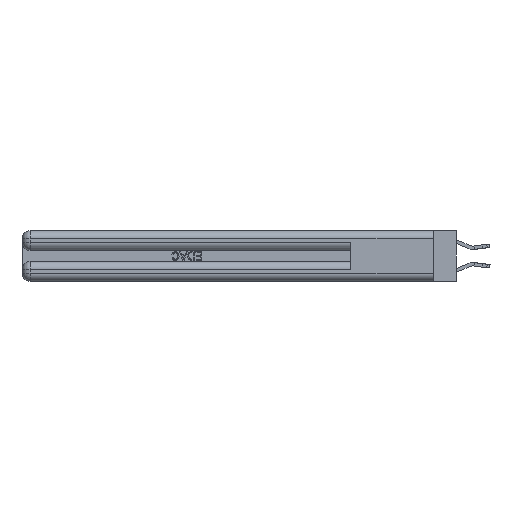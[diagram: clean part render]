
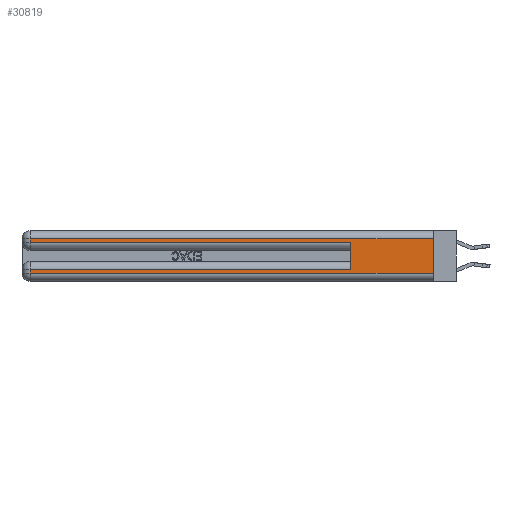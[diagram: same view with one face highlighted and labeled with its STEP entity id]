
A CAD part, left-side view. The second image highlights one B-rep face of the part: STEP entity #30819.
In plain terms, the highlighted planar face has unit normal (-1, 0, 0).
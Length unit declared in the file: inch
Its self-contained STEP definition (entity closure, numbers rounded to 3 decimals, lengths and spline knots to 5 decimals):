
#373 = EDGE_CURVE ( 'NONE', #23532, #20801, #22028, .T. ) ;
#818 = FACE_OUTER_BOUND ( 'NONE', #31482, .T. ) ;
#978 = CARTESIAN_POINT ( 'NONE',  ( 0., 0.6, 0.285 ) ) ;
#1347 = VERTEX_POINT ( 'NONE', #12245 ) ;
#1955 = DIRECTION ( 'NONE',  ( 0., 0., -1. ) ) ;
#3274 = ORIENTED_EDGE ( 'NONE', *, *, #20237, .T. ) ;
#3309 = LINE ( 'NONE', #18351, #28247 ) ;
#3530 = CARTESIAN_POINT ( 'NONE',  ( 0., 0., 0.06 ) ) ;
#5836 = VERTEX_POINT ( 'NONE', #17607 ) ;
#5898 = DIRECTION ( 'NONE',  ( 0., 1., 0. ) ) ;
#6090 = LINE ( 'NONE', #21295, #30960 ) ;
#6137 = EDGE_CURVE ( 'NONE', #17346, #1347, #9753, .T. ) ;
#6202 = CARTESIAN_POINT ( 'NONE',  ( 0., 0., 0.31 ) ) ;
#7360 = ORIENTED_EDGE ( 'NONE', *, *, #18327, .T. ) ;
#7381 = CARTESIAN_POINT ( 'NONE',  ( 0., 2.94, 0.085 ) ) ;
#7433 = CARTESIAN_POINT ( 'NONE',  ( 0., 2.94, 0.285 ) ) ;
#8751 = VECTOR ( 'NONE', #27055, 39.37008 ) ;
#8969 = ORIENTED_EDGE ( 'NONE', *, *, #12586, .T. ) ;
#9753 = LINE ( 'NONE', #19780, #20037 ) ;
#10319 = LINE ( 'NONE', #3530, #29780 ) ;
#11168 = EDGE_CURVE ( 'NONE', #29042, #22127, #17616, .T. ) ;
#11411 = CARTESIAN_POINT ( 'NONE',  ( 0., 0., 0.31 ) ) ;
#12245 = CARTESIAN_POINT ( 'NONE',  ( 0., 2.94, 0.06 ) ) ;
#12586 = EDGE_CURVE ( 'NONE', #29042, #17346, #3309, .T. ) ;
#12963 = CARTESIAN_POINT ( 'NONE',  ( 0., 0., 0.37 ) ) ;
#13452 = LINE ( 'NONE', #21529, #31425 ) ;
#13835 = ORIENTED_EDGE ( 'NONE', *, *, #30944, .T. ) ;
#14532 = CARTESIAN_POINT ( 'NONE',  ( 0., 0.6, 0.145 ) ) ;
#15173 = DIRECTION ( 'NONE',  ( 0., -1., 0. ) ) ;
#15955 = DIRECTION ( 'NONE',  ( 0., 0., -1. ) ) ;
#16271 = ORIENTED_EDGE ( 'NONE', *, *, #373, .T. ) ;
#16440 = AXIS2_PLACEMENT_3D ( 'NONE', #12963, #24951, #27383 ) ;
#17236 = ORIENTED_EDGE ( 'NONE', *, *, #31134, .F. ) ;
#17346 = VERTEX_POINT ( 'NONE', #7381 ) ;
#17607 = CARTESIAN_POINT ( 'NONE',  ( 0., 0., 0.06 ) ) ;
#17616 = LINE ( 'NONE', #14532, #25312 ) ;
#18296 = DIRECTION ( 'NONE',  ( 0., -1., 0. ) ) ;
#18327 = EDGE_CURVE ( 'NONE', #1347, #5836, #10319, .T. ) ;
#18351 = CARTESIAN_POINT ( 'NONE',  ( 0., 0., 0.085 ) ) ;
#19583 = CARTESIAN_POINT ( 'NONE',  ( 0., 0., 0.37 ) ) ;
#19780 = CARTESIAN_POINT ( 'NONE',  ( 0., 2.94, 0.37 ) ) ;
#20037 = VECTOR ( 'NONE', #29510, 39.37008 ) ;
#20237 = EDGE_CURVE ( 'NONE', #20801, #31113, #6090, .T. ) ;
#20801 = VERTEX_POINT ( 'NONE', #23303 ) ;
#21295 = CARTESIAN_POINT ( 'NONE',  ( 0., 2.94, 0.37 ) ) ;
#21529 = CARTESIAN_POINT ( 'NONE',  ( 0., 0., 0.285 ) ) ;
#21781 = ORIENTED_EDGE ( 'NONE', *, *, #6137, .T. ) ;
#22028 = LINE ( 'NONE', #11411, #8751 ) ;
#22127 = VERTEX_POINT ( 'NONE', #978 ) ;
#22449 = DIRECTION ( 'NONE',  ( 0., 0., 1. ) ) ;
#23303 = CARTESIAN_POINT ( 'NONE',  ( 0., 2.94, 0.31 ) ) ;
#23532 = VERTEX_POINT ( 'NONE', #6202 ) ;
#24507 = CARTESIAN_POINT ( 'NONE',  ( 0., 0.6, 0.085 ) ) ;
#24589 = LINE ( 'NONE', #19583, #26821 ) ;
#24951 = DIRECTION ( 'NONE',  ( 1., 0., 0. ) ) ;
#25312 = VECTOR ( 'NONE', #22449, 39.37008 ) ;
#25538 = ORIENTED_EDGE ( 'NONE', *, *, #11168, .F. ) ;
#26821 = VECTOR ( 'NONE', #1955, 39.37008 ) ;
#27055 = DIRECTION ( 'NONE',  ( 0., 1., 0. ) ) ;
#27383 = DIRECTION ( 'NONE',  ( 0., 0., -1. ) ) ;
#28247 = VECTOR ( 'NONE', #5898, 39.37008 ) ;
#29042 = VERTEX_POINT ( 'NONE', #24507 ) ;
#29510 = DIRECTION ( 'NONE',  ( 0., 0., -1. ) ) ;
#29780 = VECTOR ( 'NONE', #15173, 39.37008 ) ;
#29970 = PLANE ( 'NONE',  #16440 ) ;
#30819 = ADVANCED_FACE ( 'NONE', ( #818 ), #29970, .F. ) ;
#30944 = EDGE_CURVE ( 'NONE', #31113, #22127, #13452, .T. ) ;
#30960 = VECTOR ( 'NONE', #15955, 39.37008 ) ;
#31113 = VERTEX_POINT ( 'NONE', #7433 ) ;
#31134 = EDGE_CURVE ( 'NONE', #23532, #5836, #24589, .T. ) ;
#31425 = VECTOR ( 'NONE', #18296, 39.37008 ) ;
#31482 = EDGE_LOOP ( 'NONE', ( #17236, #16271, #3274, #13835, #25538, #8969, #21781, #7360 ) ) ;
